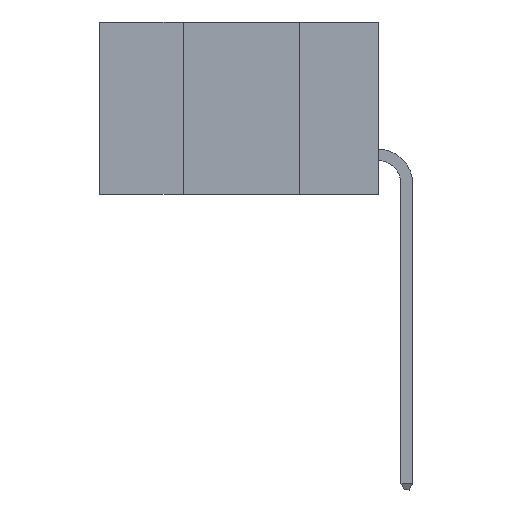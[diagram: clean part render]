
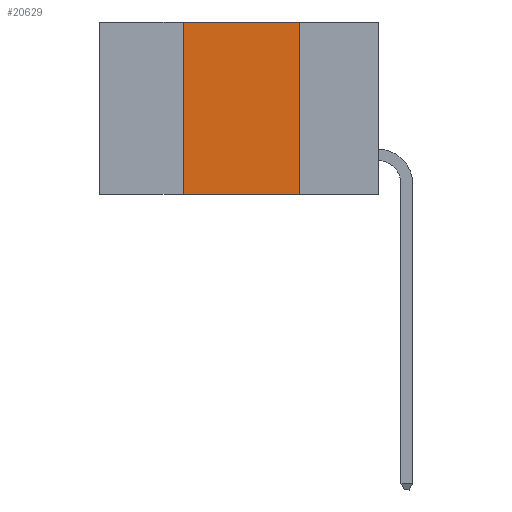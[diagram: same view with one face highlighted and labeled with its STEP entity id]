
A CAD part, left-side view. The second image highlights one B-rep face of the part: STEP entity #20629.
In plain terms, the highlighted planar face has unit normal (-1, 0, 0).
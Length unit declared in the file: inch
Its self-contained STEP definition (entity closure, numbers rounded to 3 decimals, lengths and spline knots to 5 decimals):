
#87 = VECTOR ( 'NONE', #11915, 39.37008 ) ;
#200 = LINE ( 'NONE', #16653, #7917 ) ;
#318 = DIRECTION ( 'NONE',  ( 0., 0., 1. ) ) ;
#1338 = DIRECTION ( 'NONE',  ( 0., 0., -1. ) ) ;
#2406 = VERTEX_POINT ( 'NONE', #6166 ) ;
#2700 = EDGE_CURVE ( 'NONE', #22593, #15353, #5983, .T. ) ;
#4633 = CARTESIAN_POINT ( 'NONE',  ( 0., 0.17, 0. ) ) ;
#5060 = EDGE_CURVE ( 'NONE', #17521, #2406, #20856, .T. ) ;
#5485 = CARTESIAN_POINT ( 'NONE',  ( 0., 0.6, 0. ) ) ;
#5711 = FACE_OUTER_BOUND ( 'NONE', #15177, .T. ) ;
#5983 = LINE ( 'NONE', #8946, #19257 ) ;
#6166 = CARTESIAN_POINT ( 'NONE',  ( 0., 0.17, 0. ) ) ;
#6735 = ORIENTED_EDGE ( 'NONE', *, *, #19182, .F. ) ;
#7822 = CARTESIAN_POINT ( 'NONE',  ( 0., 0.17, -0.37 ) ) ;
#7917 = VECTOR ( 'NONE', #318, 39.37008 ) ;
#8946 = CARTESIAN_POINT ( 'NONE',  ( 0., 0.6, -0.37 ) ) ;
#9577 = DIRECTION ( 'NONE',  ( 0., -1., 0. ) ) ;
#10215 = ORIENTED_EDGE ( 'NONE', *, *, #18482, .F. ) ;
#11915 = DIRECTION ( 'NONE',  ( 0., 0., -1. ) ) ;
#12201 = PLANE ( 'NONE',  #16585 ) ;
#13251 = VECTOR ( 'NONE', #15598, 39.37008 ) ;
#15177 = EDGE_LOOP ( 'NONE', ( #6735, #18309, #10215, #23231 ) ) ;
#15353 = VERTEX_POINT ( 'NONE', #7822 ) ;
#15598 = DIRECTION ( 'NONE',  ( 0., -1., 0. ) ) ;
#15911 = CARTESIAN_POINT ( 'NONE',  ( 0., 0.42, 0. ) ) ;
#15972 = LINE ( 'NONE', #4633, #87 ) ;
#16585 = AXIS2_PLACEMENT_3D ( 'NONE', #5485, #18156, #1338 ) ;
#16653 = CARTESIAN_POINT ( 'NONE',  ( 0., 0.42, 0. ) ) ;
#17521 = VERTEX_POINT ( 'NONE', #15911 ) ;
#18156 = DIRECTION ( 'NONE',  ( 1., 0., 0. ) ) ;
#18309 = ORIENTED_EDGE ( 'NONE', *, *, #5060, .F. ) ;
#18482 = EDGE_CURVE ( 'NONE', #22593, #17521, #200, .T. ) ;
#19182 = EDGE_CURVE ( 'NONE', #2406, #15353, #15972, .T. ) ;
#19226 = CARTESIAN_POINT ( 'NONE',  ( 0., 0.6, 0. ) ) ;
#19257 = VECTOR ( 'NONE', #9577, 39.37008 ) ;
#20629 = ADVANCED_FACE ( 'NONE', ( #5711 ), #12201, .F. ) ;
#20856 = LINE ( 'NONE', #19226, #13251 ) ;
#21240 = CARTESIAN_POINT ( 'NONE',  ( 0., 0.42, -0.37 ) ) ;
#22593 = VERTEX_POINT ( 'NONE', #21240 ) ;
#23231 = ORIENTED_EDGE ( 'NONE', *, *, #2700, .T. ) ;
